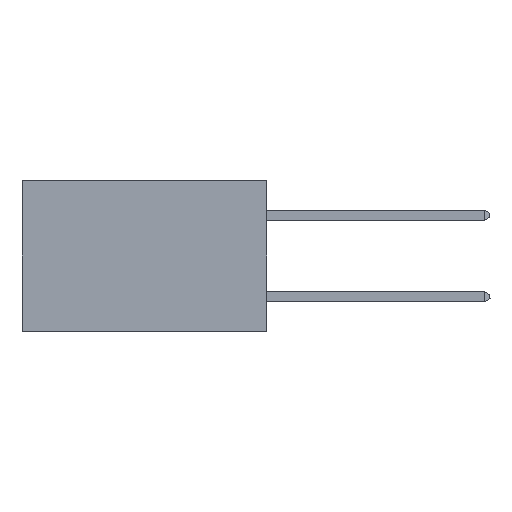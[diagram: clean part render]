
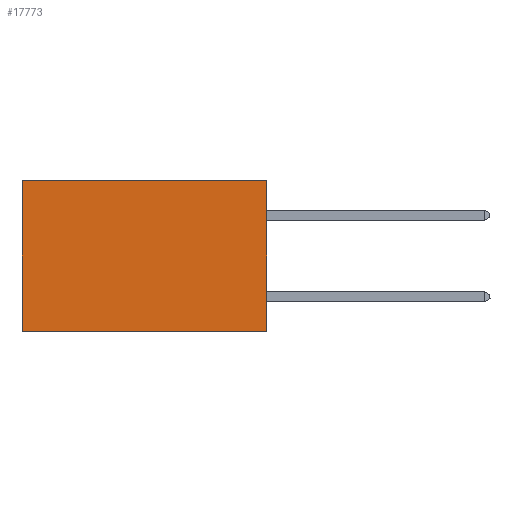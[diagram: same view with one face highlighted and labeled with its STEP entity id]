
A CAD part, left-side view. The second image highlights one B-rep face of the part: STEP entity #17773.
In plain terms, the highlighted planar face has unit normal (-1, 0, 0).
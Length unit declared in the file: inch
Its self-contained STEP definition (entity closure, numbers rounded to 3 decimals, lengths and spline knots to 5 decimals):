
#79 = ORIENTED_EDGE ( 'NONE', *, *, #22628, .T. ) ;
#538 = VECTOR ( 'NONE', #21214, 39.37008 ) ;
#582 = EDGE_CURVE ( 'NONE', #19737, #915, #9103, .T. ) ;
#915 = VERTEX_POINT ( 'NONE', #11677 ) ;
#1229 = DIRECTION ( 'NONE',  ( 1., 0., 0. ) ) ;
#1577 = EDGE_CURVE ( 'NONE', #19737, #4927, #4640, .T. ) ;
#1635 = VECTOR ( 'NONE', #18510, 39.37008 ) ;
#2743 = ORIENTED_EDGE ( 'NONE', *, *, #582, .T. ) ;
#3389 = AXIS2_PLACEMENT_3D ( 'NONE', #20826, #1229, #18945 ) ;
#4188 = DIRECTION ( 'NONE',  ( 0., 0., -1. ) ) ;
#4640 = LINE ( 'NONE', #18254, #22928 ) ;
#4927 = VERTEX_POINT ( 'NONE', #15417 ) ;
#6075 = CARTESIAN_POINT ( 'NONE',  ( 0.2875, 0., 0. ) ) ;
#6664 = LINE ( 'NONE', #8974, #538 ) ;
#7370 = CARTESIAN_POINT ( 'NONE',  ( 0.2875, 0.6, -0.37 ) ) ;
#8974 = CARTESIAN_POINT ( 'NONE',  ( 0.2875, 0., -0.37 ) ) ;
#9103 = LINE ( 'NONE', #16098, #1635 ) ;
#9429 = ORIENTED_EDGE ( 'NONE', *, *, #17447, .F. ) ;
#10990 = EDGE_LOOP ( 'NONE', ( #79, #9429, #16200, #2743 ) ) ;
#11677 = CARTESIAN_POINT ( 'NONE',  ( 0.2875, 0.6, 0. ) ) ;
#11872 = VECTOR ( 'NONE', #20281, 39.37008 ) ;
#14635 = VERTEX_POINT ( 'NONE', #7370 ) ;
#15417 = CARTESIAN_POINT ( 'NONE',  ( 0.2875, 0., -0.37 ) ) ;
#16098 = CARTESIAN_POINT ( 'NONE',  ( 0.2875, 0., 0. ) ) ;
#16200 = ORIENTED_EDGE ( 'NONE', *, *, #1577, .F. ) ;
#16314 = LINE ( 'NONE', #18475, #11872 ) ;
#16573 = FACE_OUTER_BOUND ( 'NONE', #10990, .T. ) ;
#17447 = EDGE_CURVE ( 'NONE', #4927, #14635, #6664, .T. ) ;
#17773 = ADVANCED_FACE ( 'NONE', ( #16573 ), #19012, .F. ) ;
#18254 = CARTESIAN_POINT ( 'NONE',  ( 0.2875, 0., 0. ) ) ;
#18475 = CARTESIAN_POINT ( 'NONE',  ( 0.2875, 0.6, 0. ) ) ;
#18510 = DIRECTION ( 'NONE',  ( 0., 1., 0. ) ) ;
#18945 = DIRECTION ( 'NONE',  ( 0., 0., -1. ) ) ;
#19012 = PLANE ( 'NONE',  #3389 ) ;
#19737 = VERTEX_POINT ( 'NONE', #6075 ) ;
#20281 = DIRECTION ( 'NONE',  ( 0., 0., -1. ) ) ;
#20826 = CARTESIAN_POINT ( 'NONE',  ( 0.2875, 0., 0. ) ) ;
#21214 = DIRECTION ( 'NONE',  ( 0., 1., 0. ) ) ;
#22628 = EDGE_CURVE ( 'NONE', #915, #14635, #16314, .T. ) ;
#22928 = VECTOR ( 'NONE', #4188, 39.37008 ) ;
